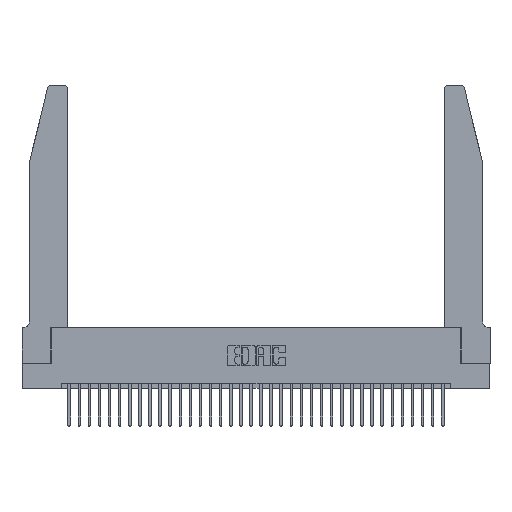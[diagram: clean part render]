
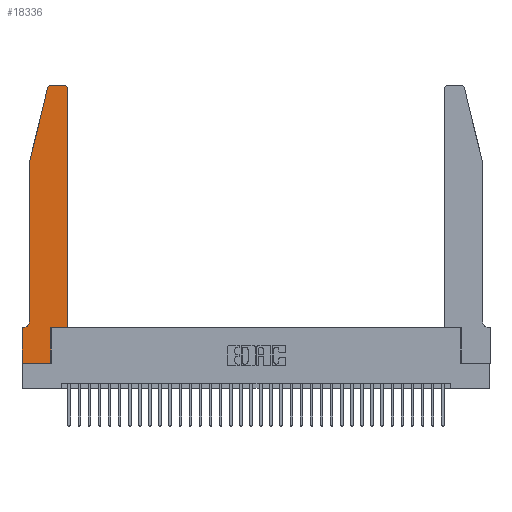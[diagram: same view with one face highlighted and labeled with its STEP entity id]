
A CAD part, top view. The second image highlights one B-rep face of the part: STEP entity #18336.
In plain terms, the highlighted planar face has unit normal (0, 0, 1).
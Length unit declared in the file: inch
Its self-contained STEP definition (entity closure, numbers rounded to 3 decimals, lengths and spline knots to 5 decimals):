
#183 = CARTESIAN_POINT ( 'NONE',  ( 0.0755, 0.42, 0.37 ) ) ;
#705 = AXIS2_PLACEMENT_3D ( 'NONE', #14952, #33655, #17676 ) ;
#744 = EDGE_CURVE ( 'NONE', #20630, #32939, #7388, .T. ) ;
#1125 = ORIENTED_EDGE ( 'NONE', *, *, #23884, .T. ) ;
#2370 = EDGE_LOOP ( 'NONE', ( #10949, #32372, #8981, #22174, #1125, #3004, #18904, #6527, #31431, #14104, #8262, #5095 ) ) ;
#2396 = DIRECTION ( 'NONE',  ( 1., 0., 0. ) ) ;
#2586 = DIRECTION ( 'NONE',  ( 0., 1., 0. ) ) ;
#3004 = ORIENTED_EDGE ( 'NONE', *, *, #32948, .T. ) ;
#3584 = CIRCLE ( 'NONE', #6403, 0.07 ) ;
#3988 = VERTEX_POINT ( 'NONE', #14192 ) ;
#4295 = EDGE_CURVE ( 'NONE', #29953, #26326, #26928, .T. ) ;
#4617 = VERTEX_POINT ( 'NONE', #183 ) ;
#5095 = ORIENTED_EDGE ( 'NONE', *, *, #744, .T. ) ;
#5144 = LINE ( 'NONE', #33390, #18827 ) ;
#6403 = AXIS2_PLACEMENT_3D ( 'NONE', #27076, #10940, #29774 ) ;
#6527 = ORIENTED_EDGE ( 'NONE', *, *, #16865, .T. ) ;
#6735 = CARTESIAN_POINT ( 'NONE',  ( 0.4205, 2.72, 0.37 ) ) ;
#7388 = CIRCLE ( 'NONE', #24827, 0.03 ) ;
#7591 = DIRECTION ( 'NONE',  ( 0., -1., 0. ) ) ;
#8204 = CARTESIAN_POINT ( 'NONE',  ( 0.2865, 0., 0.37 ) ) ;
#8262 = ORIENTED_EDGE ( 'NONE', *, *, #31671, .T. ) ;
#8281 = EDGE_CURVE ( 'NONE', #3988, #14726, #25859, .T. ) ;
#8446 = CARTESIAN_POINT ( 'NONE',  ( 0., 0., 0.37 ) ) ;
#8736 = VERTEX_POINT ( 'NONE', #17004 ) ;
#8981 = ORIENTED_EDGE ( 'NONE', *, *, #28223, .T. ) ;
#9494 = DIRECTION ( 'NONE',  ( 1., 0., 0. ) ) ;
#9650 = LINE ( 'NONE', #15903, #23255 ) ;
#9855 = VECTOR ( 'NONE', #2586, 39.37008 ) ;
#9912 = VECTOR ( 'NONE', #2396, 39.37008 ) ;
#10042 = EDGE_CURVE ( 'NONE', #8736, #30848, #30598, .T. ) ;
#10453 = CARTESIAN_POINT ( 'NONE',  ( 0.2605, 2.75, 0.37 ) ) ;
#10940 = DIRECTION ( 'NONE',  ( 0., 0., -1. ) ) ;
#10949 = ORIENTED_EDGE ( 'NONE', *, *, #34217, .T. ) ;
#11502 = LINE ( 'NONE', #31710, #31276 ) ;
#11521 = VECTOR ( 'NONE', #20068, 39.37008 ) ;
#12763 = CARTESIAN_POINT ( 'NONE',  ( 0.4505, 0.35, 0.37 ) ) ;
#13559 = CARTESIAN_POINT ( 'NONE',  ( 0.0055, 0.35, 0.37 ) ) ;
#13733 = CARTESIAN_POINT ( 'NONE',  ( 0.0755, 0.35, 0.37 ) ) ;
#14104 = ORIENTED_EDGE ( 'NONE', *, *, #10042, .T. ) ;
#14192 = CARTESIAN_POINT ( 'NONE',  ( 0., 0.35, 0.37 ) ) ;
#14508 = VECTOR ( 'NONE', #26639, 39.37008 ) ;
#14709 = EDGE_CURVE ( 'NONE', #30508, #8736, #17392, .T. ) ;
#14726 = VERTEX_POINT ( 'NONE', #8446 ) ;
#14877 = CARTESIAN_POINT ( 'NONE',  ( 0.284, 2.75, 0.37 ) ) ;
#14952 = CARTESIAN_POINT ( 'NONE',  ( 0., 0.35, 0.37 ) ) ;
#15340 = DIRECTION ( 'NONE',  ( 0., 0., 1. ) ) ;
#15903 = CARTESIAN_POINT ( 'NONE',  ( 0.0755, 2., 0.37 ) ) ;
#16619 = DIRECTION ( 'NONE',  ( 0., 1., 0. ) ) ;
#16756 = VERTEX_POINT ( 'NONE', #30268 ) ;
#16865 = EDGE_CURVE ( 'NONE', #14726, #30508, #5144, .T. ) ;
#17004 = CARTESIAN_POINT ( 'NONE',  ( 0.2865, 0.35, 0.37 ) ) ;
#17392 = LINE ( 'NONE', #32622, #30750 ) ;
#17676 = DIRECTION ( 'NONE',  ( 1., 0., 0. ) ) ;
#18336 = ADVANCED_FACE ( 'NONE', ( #21649 ), #30975, .T. ) ;
#18827 = VECTOR ( 'NONE', #30721, 39.37008 ) ;
#18904 = ORIENTED_EDGE ( 'NONE', *, *, #8281, .T. ) ;
#19165 = DIRECTION ( 'NONE',  ( -1., 0., 0. ) ) ;
#19342 = VERTEX_POINT ( 'NONE', #13559 ) ;
#19608 = LINE ( 'NONE', #13733, #32968 ) ;
#19740 = EDGE_CURVE ( 'NONE', #16756, #4617, #9650, .T. ) ;
#20068 = DIRECTION ( 'NONE',  ( 0., -1., 0. ) ) ;
#20630 = VERTEX_POINT ( 'NONE', #32802 ) ;
#21523 = CARTESIAN_POINT ( 'NONE',  ( 0.4505, 0.35, 0.37 ) ) ;
#21621 = CARTESIAN_POINT ( 'NONE',  ( 0.4205, 2.75, 0.37 ) ) ;
#21649 = FACE_OUTER_BOUND ( 'NONE', #2370, .T. ) ;
#21789 = AXIS2_PLACEMENT_3D ( 'NONE', #31365, #15340, #34036 ) ;
#22174 = ORIENTED_EDGE ( 'NONE', *, *, #19740, .T. ) ;
#23255 = VECTOR ( 'NONE', #7591, 39.37008 ) ;
#23787 = DIRECTION ( 'NONE',  ( -0.239, -0.971, 0. ) ) ;
#23884 = EDGE_CURVE ( 'NONE', #4617, #19342, #3584, .T. ) ;
#24289 = LINE ( 'NONE', #32315, #9855 ) ;
#24827 = AXIS2_PLACEMENT_3D ( 'NONE', #6735, #25708, #9494 ) ;
#25099 = CARTESIAN_POINT ( 'NONE',  ( 0.25487, 2.72718, 0.37 ) ) ;
#25708 = DIRECTION ( 'NONE',  ( 0., 0., 1. ) ) ;
#25859 = LINE ( 'NONE', #33359, #11521 ) ;
#26326 = VERTEX_POINT ( 'NONE', #25099 ) ;
#26639 = DIRECTION ( 'NONE',  ( -1., 0., 0. ) ) ;
#26928 = CIRCLE ( 'NONE', #21789, 0.03 ) ;
#27076 = CARTESIAN_POINT ( 'NONE',  ( 0.0055, 0.42, 0.37 ) ) ;
#28223 = EDGE_CURVE ( 'NONE', #26326, #16756, #11502, .T. ) ;
#29774 = DIRECTION ( 'NONE',  ( -1., 0., 0. ) ) ;
#29953 = VERTEX_POINT ( 'NONE', #14877 ) ;
#30268 = CARTESIAN_POINT ( 'NONE',  ( 0.0755, 2., 0.37 ) ) ;
#30415 = LINE ( 'NONE', #10453, #14508 ) ;
#30508 = VERTEX_POINT ( 'NONE', #8204 ) ;
#30598 = LINE ( 'NONE', #21523, #9912 ) ;
#30721 = DIRECTION ( 'NONE',  ( 1., 0., 0. ) ) ;
#30750 = VECTOR ( 'NONE', #16619, 39.37008 ) ;
#30848 = VERTEX_POINT ( 'NONE', #12763 ) ;
#30975 = PLANE ( 'NONE',  #705 ) ;
#31276 = VECTOR ( 'NONE', #23787, 39.37008 ) ;
#31365 = CARTESIAN_POINT ( 'NONE',  ( 0.284, 2.72, 0.37 ) ) ;
#31431 = ORIENTED_EDGE ( 'NONE', *, *, #14709, .T. ) ;
#31671 = EDGE_CURVE ( 'NONE', #30848, #20630, #24289, .T. ) ;
#31710 = CARTESIAN_POINT ( 'NONE',  ( 0.0755, 2., 0.37 ) ) ;
#32315 = CARTESIAN_POINT ( 'NONE',  ( 0.4505, 0.35, 0.37 ) ) ;
#32372 = ORIENTED_EDGE ( 'NONE', *, *, #4295, .T. ) ;
#32622 = CARTESIAN_POINT ( 'NONE',  ( 0.2865, 0.35, 0.37 ) ) ;
#32802 = CARTESIAN_POINT ( 'NONE',  ( 0.4505, 2.72, 0.37 ) ) ;
#32939 = VERTEX_POINT ( 'NONE', #21621 ) ;
#32948 = EDGE_CURVE ( 'NONE', #19342, #3988, #19608, .T. ) ;
#32968 = VECTOR ( 'NONE', #19165, 39.37008 ) ;
#33359 = CARTESIAN_POINT ( 'NONE',  ( 0., 0., 0.37 ) ) ;
#33390 = CARTESIAN_POINT ( 'NONE',  ( 0., 0., 0.37 ) ) ;
#33655 = DIRECTION ( 'NONE',  ( 0., 0., 1. ) ) ;
#34036 = DIRECTION ( 'NONE',  ( 1., 0., 0. ) ) ;
#34217 = EDGE_CURVE ( 'NONE', #32939, #29953, #30415, .T. ) ;
